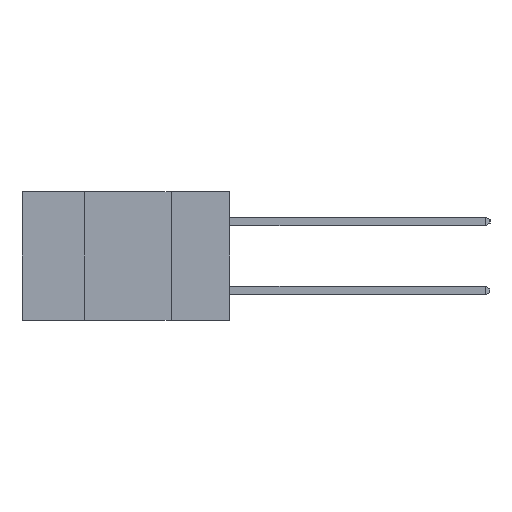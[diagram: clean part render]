
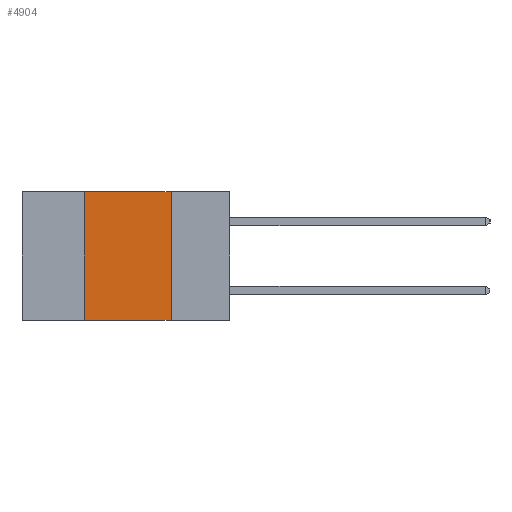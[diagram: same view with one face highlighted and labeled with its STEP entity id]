
A CAD part, left-side view. The second image highlights one B-rep face of the part: STEP entity #4904.
In plain terms, the highlighted planar face has unit normal (-1, 0, 0).
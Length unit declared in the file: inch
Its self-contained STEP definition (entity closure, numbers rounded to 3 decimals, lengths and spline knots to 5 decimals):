
#17 = VECTOR ( 'NONE', #4366, 39.37008 ) ;
#85 = DIRECTION ( 'NONE',  ( 1., 0., 0. ) ) ;
#135 = LINE ( 'NONE', #7637, #2505 ) ;
#323 = LINE ( 'NONE', #6341, #17 ) ;
#541 = EDGE_LOOP ( 'NONE', ( #6795, #3087, #8966, #730 ) ) ;
#598 = CARTESIAN_POINT ( 'NONE',  ( 0., 0.6, -0.37 ) ) ;
#714 = EDGE_CURVE ( 'NONE', #6534, #1313, #900, .T. ) ;
#730 = ORIENTED_EDGE ( 'NONE', *, *, #714, .T. ) ;
#813 = EDGE_CURVE ( 'NONE', #6060, #3679, #323, .T. ) ;
#900 = LINE ( 'NONE', #598, #9188 ) ;
#1009 = LINE ( 'NONE', #6667, #2765 ) ;
#1313 = VERTEX_POINT ( 'NONE', #4649 ) ;
#2041 = EDGE_CURVE ( 'NONE', #6534, #6060, #135, .T. ) ;
#2209 = AXIS2_PLACEMENT_3D ( 'NONE', #9797, #85, #6005 ) ;
#2505 = VECTOR ( 'NONE', #7557, 39.37008 ) ;
#2765 = VECTOR ( 'NONE', #7276, 39.37008 ) ;
#3087 = ORIENTED_EDGE ( 'NONE', *, *, #813, .F. ) ;
#3194 = EDGE_CURVE ( 'NONE', #3679, #1313, #1009, .T. ) ;
#3679 = VERTEX_POINT ( 'NONE', #7573 ) ;
#3898 = DIRECTION ( 'NONE',  ( 0., -1., 0. ) ) ;
#4366 = DIRECTION ( 'NONE',  ( 0., -1., 0. ) ) ;
#4649 = CARTESIAN_POINT ( 'NONE',  ( 0., 0.17, -0.37 ) ) ;
#4904 = ADVANCED_FACE ( 'NONE', ( #7918 ), #8982, .F. ) ;
#6005 = DIRECTION ( 'NONE',  ( 0., 0., -1. ) ) ;
#6060 = VERTEX_POINT ( 'NONE', #6615 ) ;
#6341 = CARTESIAN_POINT ( 'NONE',  ( 0., 0.6, 0. ) ) ;
#6534 = VERTEX_POINT ( 'NONE', #9597 ) ;
#6615 = CARTESIAN_POINT ( 'NONE',  ( 0., 0.42, 0. ) ) ;
#6667 = CARTESIAN_POINT ( 'NONE',  ( 0., 0.17, 0. ) ) ;
#6795 = ORIENTED_EDGE ( 'NONE', *, *, #3194, .F. ) ;
#7276 = DIRECTION ( 'NONE',  ( 0., 0., -1. ) ) ;
#7557 = DIRECTION ( 'NONE',  ( 0., 0., 1. ) ) ;
#7573 = CARTESIAN_POINT ( 'NONE',  ( 0., 0.17, 0. ) ) ;
#7637 = CARTESIAN_POINT ( 'NONE',  ( 0., 0.42, 0. ) ) ;
#7918 = FACE_OUTER_BOUND ( 'NONE', #541, .T. ) ;
#8966 = ORIENTED_EDGE ( 'NONE', *, *, #2041, .F. ) ;
#8982 = PLANE ( 'NONE',  #2209 ) ;
#9188 = VECTOR ( 'NONE', #3898, 39.37008 ) ;
#9597 = CARTESIAN_POINT ( 'NONE',  ( 0., 0.42, -0.37 ) ) ;
#9797 = CARTESIAN_POINT ( 'NONE',  ( 0., 0.6, 0. ) ) ;
